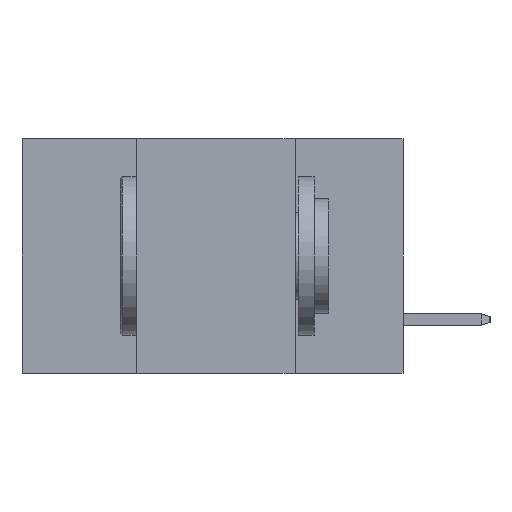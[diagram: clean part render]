
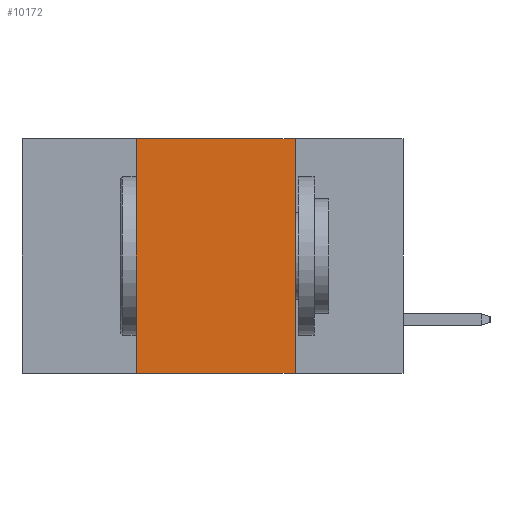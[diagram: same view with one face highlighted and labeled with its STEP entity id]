
A CAD part, left-side view. The second image highlights one B-rep face of the part: STEP entity #10172.
In plain terms, the highlighted planar face has unit normal (-1, 0, 0).
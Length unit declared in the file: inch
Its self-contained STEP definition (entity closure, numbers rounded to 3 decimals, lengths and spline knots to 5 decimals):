
#598 = VERTEX_POINT ( 'NONE', #6950 ) ;
#836 = DIRECTION ( 'NONE',  ( 1., 0., 0. ) ) ;
#969 = AXIS2_PLACEMENT_3D ( 'NONE', #7557, #836, #6721 ) ;
#1524 = ORIENTED_EDGE ( 'NONE', *, *, #9585, .T. ) ;
#1691 = CARTESIAN_POINT ( 'NONE',  ( 0., 0.17, 0. ) ) ;
#1745 = VECTOR ( 'NONE', #4872, 39.37008 ) ;
#1820 = VECTOR ( 'NONE', #6609, 39.37008 ) ;
#2762 = FACE_OUTER_BOUND ( 'NONE', #6847, .T. ) ;
#3563 = CARTESIAN_POINT ( 'NONE',  ( 0., 0.17, 0. ) ) ;
#3623 = EDGE_CURVE ( 'NONE', #5245, #3789, #4770, .T. ) ;
#3789 = VERTEX_POINT ( 'NONE', #11401 ) ;
#4353 = VERTEX_POINT ( 'NONE', #3563 ) ;
#4770 = LINE ( 'NONE', #5616, #1820 ) ;
#4872 = DIRECTION ( 'NONE',  ( 0., -1., 0. ) ) ;
#5116 = EDGE_CURVE ( 'NONE', #4353, #598, #8676, .T. ) ;
#5215 = CARTESIAN_POINT ( 'NONE',  ( 0., 0.6, 0. ) ) ;
#5245 = VERTEX_POINT ( 'NONE', #5357 ) ;
#5357 = CARTESIAN_POINT ( 'NONE',  ( 0., 0.42, -0.37 ) ) ;
#5616 = CARTESIAN_POINT ( 'NONE',  ( 0., 0.42, 0. ) ) ;
#6609 = DIRECTION ( 'NONE',  ( 0., 0., 1. ) ) ;
#6721 = DIRECTION ( 'NONE',  ( 0., 0., -1. ) ) ;
#6847 = EDGE_LOOP ( 'NONE', ( #11703, #12377, #8071, #1524 ) ) ;
#6950 = CARTESIAN_POINT ( 'NONE',  ( 0., 0.17, -0.37 ) ) ;
#7557 = CARTESIAN_POINT ( 'NONE',  ( 0., 0.6, 0. ) ) ;
#8071 = ORIENTED_EDGE ( 'NONE', *, *, #3623, .F. ) ;
#8676 = LINE ( 'NONE', #1691, #12357 ) ;
#9133 = CARTESIAN_POINT ( 'NONE',  ( 0., 0.6, -0.37 ) ) ;
#9281 = EDGE_CURVE ( 'NONE', #3789, #4353, #10308, .T. ) ;
#9380 = VECTOR ( 'NONE', #12033, 39.37008 ) ;
#9585 = EDGE_CURVE ( 'NONE', #5245, #598, #10743, .T. ) ;
#10172 = ADVANCED_FACE ( 'NONE', ( #2762 ), #10450, .F. ) ;
#10308 = LINE ( 'NONE', #5215, #9380 ) ;
#10450 = PLANE ( 'NONE',  #969 ) ;
#10743 = LINE ( 'NONE', #9133, #1745 ) ;
#11401 = CARTESIAN_POINT ( 'NONE',  ( 0., 0.42, 0. ) ) ;
#11703 = ORIENTED_EDGE ( 'NONE', *, *, #5116, .F. ) ;
#12033 = DIRECTION ( 'NONE',  ( 0., -1., 0. ) ) ;
#12357 = VECTOR ( 'NONE', #12632, 39.37008 ) ;
#12377 = ORIENTED_EDGE ( 'NONE', *, *, #9281, .F. ) ;
#12632 = DIRECTION ( 'NONE',  ( 0., 0., -1. ) ) ;
